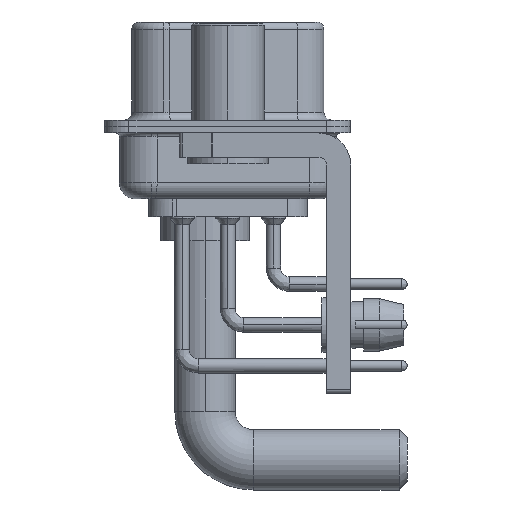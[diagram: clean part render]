
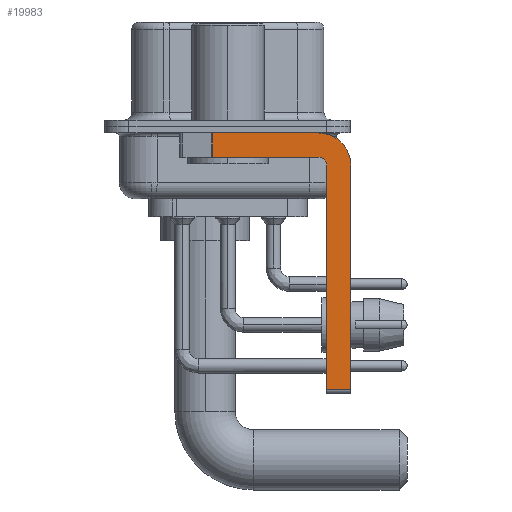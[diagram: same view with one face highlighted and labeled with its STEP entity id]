
A CAD part, left-side view. The second image highlights one B-rep face of the part: STEP entity #19983.
In plain terms, the highlighted planar face has unit normal (-1, 0, 0).
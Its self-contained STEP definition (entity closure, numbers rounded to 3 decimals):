
#82 = VERTEX_POINT ( 'NONE', #7500 ) ;
#563 = LINE ( 'NONE', #6979, #18899 ) ;
#1230 = FACE_OUTER_BOUND ( 'NONE', #7460, .T. ) ;
#1281 = CARTESIAN_POINT ( 'NONE',  ( -2.9, -5.65, -0.4 ) ) ;
#1985 = LINE ( 'NONE', #27256, #27426 ) ;
#2194 = CIRCLE ( 'NONE', #34603, 0.5 ) ;
#2533 = AXIS2_PLACEMENT_3D ( 'NONE', #19684, #36214, #19883 ) ;
#4847 = EDGE_CURVE ( 'NONE', #29161, #82, #29676, .T. ) ;
#4891 = DIRECTION ( 'NONE',  ( 0., 0., -1. ) ) ;
#6979 = CARTESIAN_POINT ( 'NONE',  ( -2.9, -5.65, -1.9 ) ) ;
#7002 = ORIENTED_EDGE ( 'NONE', *, *, #10323, .F. ) ;
#7460 = EDGE_LOOP ( 'NONE', ( #25960, #17483, #31737, #7002, #23920, #14615, #30772, #36126 ) ) ;
#7500 = CARTESIAN_POINT ( 'NONE',  ( -2.9, -7.65, -2.4 ) ) ;
#7844 = AXIS2_PLACEMENT_3D ( 'NONE', #14819, #40077, #30972 ) ;
#9302 = CARTESIAN_POINT ( 'NONE',  ( -2.9, -6.15, -16.35 ) ) ;
#10323 = EDGE_CURVE ( 'NONE', #32644, #24862, #2194, .T. ) ;
#10650 = EDGE_CURVE ( 'NONE', #39846, #32644, #13604, .T. ) ;
#11335 = CARTESIAN_POINT ( 'NONE',  ( -2.9, -5.65, -16.35 ) ) ;
#12576 = DIRECTION ( 'NONE',  ( 0., 0., -1. ) ) ;
#13341 = EDGE_CURVE ( 'NONE', #21240, #29161, #24988, .T. ) ;
#13604 = LINE ( 'NONE', #23747, #17442 ) ;
#14615 = ORIENTED_EDGE ( 'NONE', *, *, #25799, .T. ) ;
#14819 = CARTESIAN_POINT ( 'NONE',  ( -2.9, -5.65, -2.4 ) ) ;
#15391 = CARTESIAN_POINT ( 'NONE',  ( -2.9, -7.65, -16.35 ) ) ;
#15662 = DIRECTION ( 'NONE',  ( 0., -1., 0. ) ) ;
#17442 = VECTOR ( 'NONE', #29546, 1000. ) ;
#17483 = ORIENTED_EDGE ( 'NONE', *, *, #34193, .T. ) ;
#17736 = CARTESIAN_POINT ( 'NONE',  ( -2.9, 0.978, -1.9 ) ) ;
#18880 = VECTOR ( 'NONE', #12576, 1000. ) ;
#18899 = VECTOR ( 'NONE', #38056, 1000. ) ;
#19684 = CARTESIAN_POINT ( 'NONE',  ( -2.9, -5.65, -2.4 ) ) ;
#19745 = CARTESIAN_POINT ( 'NONE',  ( -2.9, -5.65, -1.9 ) ) ;
#19883 = DIRECTION ( 'NONE',  ( 0., 0., -1. ) ) ;
#19983 = ADVANCED_FACE ( 'NONE', ( #1230 ), #35605, .F. ) ;
#20123 = DIRECTION ( 'NONE',  ( -1., 0., 0. ) ) ;
#20172 = LINE ( 'NONE', #37607, #18880 ) ;
#20176 = CARTESIAN_POINT ( 'NONE',  ( -2.9, -6.15, -2.4 ) ) ;
#21240 = VERTEX_POINT ( 'NONE', #26918 ) ;
#22090 = CARTESIAN_POINT ( 'NONE',  ( -2.9, 3., -0.4 ) ) ;
#23747 = CARTESIAN_POINT ( 'NONE',  ( -2.9, -6.15, -16.6 ) ) ;
#23920 = ORIENTED_EDGE ( 'NONE', *, *, #10650, .F. ) ;
#24862 = VERTEX_POINT ( 'NONE', #19745 ) ;
#24988 = LINE ( 'NONE', #22090, #34589 ) ;
#25799 = EDGE_CURVE ( 'NONE', #39846, #32798, #27273, .T. ) ;
#25960 = ORIENTED_EDGE ( 'NONE', *, *, #13341, .F. ) ;
#26540 = CARTESIAN_POINT ( 'NONE',  ( -2.9, -5.65, -2.4 ) ) ;
#26918 = CARTESIAN_POINT ( 'NONE',  ( -2.9, 0.978, -0.4 ) ) ;
#27256 = CARTESIAN_POINT ( 'NONE',  ( -2.9, 0.978, -1.9 ) ) ;
#27273 = LINE ( 'NONE', #11335, #31027 ) ;
#27426 = VECTOR ( 'NONE', #4891, 1000. ) ;
#29161 = VERTEX_POINT ( 'NONE', #1281 ) ;
#29546 = DIRECTION ( 'NONE',  ( 0., 0., 1. ) ) ;
#29676 = CIRCLE ( 'NONE', #7844, 2. ) ;
#30772 = ORIENTED_EDGE ( 'NONE', *, *, #40456, .F. ) ;
#30972 = DIRECTION ( 'NONE',  ( 0., 0., -1. ) ) ;
#31027 = VECTOR ( 'NONE', #39904, 1000. ) ;
#31737 = ORIENTED_EDGE ( 'NONE', *, *, #35167, .F. ) ;
#32644 = VERTEX_POINT ( 'NONE', #20176 ) ;
#32752 = DIRECTION ( 'NONE',  ( 0., 0., 1. ) ) ;
#32798 = VERTEX_POINT ( 'NONE', #15391 ) ;
#34193 = EDGE_CURVE ( 'NONE', #21240, #36790, #1985, .T. ) ;
#34589 = VECTOR ( 'NONE', #15662, 1000. ) ;
#34603 = AXIS2_PLACEMENT_3D ( 'NONE', #26540, #20123, #32752 ) ;
#35167 = EDGE_CURVE ( 'NONE', #24862, #36790, #563, .T. ) ;
#35605 = PLANE ( 'NONE',  #2533 ) ;
#36126 = ORIENTED_EDGE ( 'NONE', *, *, #4847, .F. ) ;
#36214 = DIRECTION ( 'NONE',  ( 1., 0., 0. ) ) ;
#36790 = VERTEX_POINT ( 'NONE', #17736 ) ;
#37607 = CARTESIAN_POINT ( 'NONE',  ( -2.9, -7.65, -2.4 ) ) ;
#38056 = DIRECTION ( 'NONE',  ( 0., 1., 0. ) ) ;
#39846 = VERTEX_POINT ( 'NONE', #9302 ) ;
#39904 = DIRECTION ( 'NONE',  ( 0., -1., 0. ) ) ;
#40077 = DIRECTION ( 'NONE',  ( 1., 0., 0. ) ) ;
#40456 = EDGE_CURVE ( 'NONE', #82, #32798, #20172, .T. ) ;
